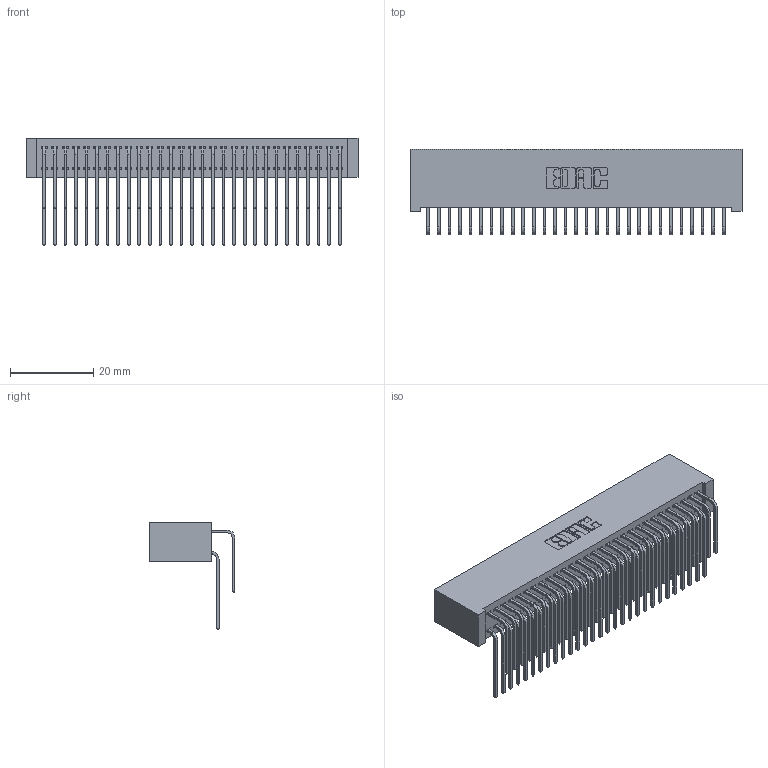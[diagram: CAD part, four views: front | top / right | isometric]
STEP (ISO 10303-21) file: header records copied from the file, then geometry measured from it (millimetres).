
FILE_DESCRIPTION (( 'STEP AP203' ), '1' );
FILE_NAME ('392-058-559-201.STEP', '2019-10-08T17:04:26', ( '' ), ( '' ), 'SwSTEP 2.0', 'SolidWorks 2016', '' );
FILE_SCHEMA (( 'CONFIG_CONTROL_DESIGN' ));
Length unit declared in the file: inch
Products named in the file (4): 392-058-559-201; 342 Part_Lugless; 345-292-001_558 559 Tail - 1; 345-292-001_559 Tail - 2
Assembly tree (59 placements, depth 2):
  392-058-559-201
    342 Part_Lugless
    345-292-001_558 559 Tail - 1  x29
    345-292-001_559 Tail - 2  x29
Bounding box: 79.91 x 20.64 x 25.78 mm (x, y, z)
Volume: 7892.3 mm3; surface area: 14486.2 mm2
Topology: 59 solids, 59 shells, 3234 faces, 9613 edges, 6330 vertices
Faces by surface type: plane 2266, cylinder 968
Entity records: 21713 total; most frequent: CARTESIAN_POINT 3661, ORIENTED_EDGE 3546, DIRECTION 3125, EDGE_CURVE 1773, LINE 1613, VECTOR 1613, VERTEX_POINT 1178, AXIS2_PLACEMENT_3D 756
